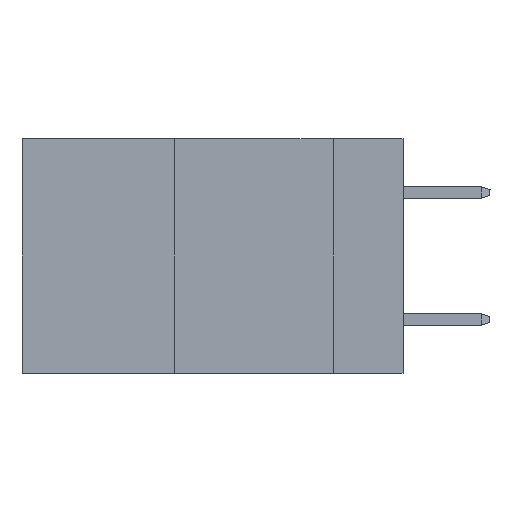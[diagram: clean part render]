
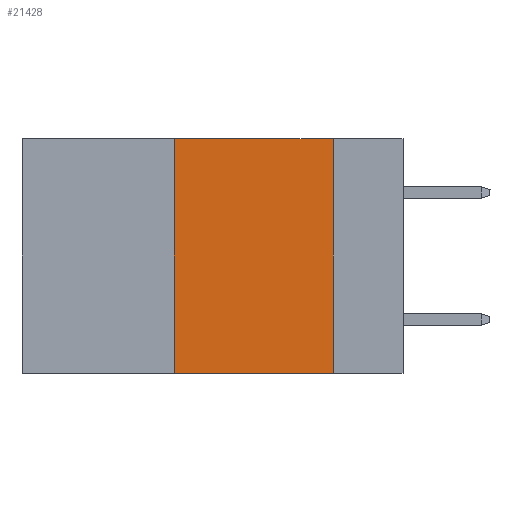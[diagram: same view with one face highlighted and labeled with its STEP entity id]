
A CAD part, left-side view. The second image highlights one B-rep face of the part: STEP entity #21428.
In plain terms, the highlighted planar face has unit normal (-1, 0, 0).
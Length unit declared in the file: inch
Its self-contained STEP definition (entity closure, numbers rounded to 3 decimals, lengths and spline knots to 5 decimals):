
#2972 = VERTEX_POINT ( 'NONE', #30787 ) ;
#3745 = VERTEX_POINT ( 'NONE', #15633 ) ;
#4530 = CARTESIAN_POINT ( 'NONE',  ( 0., 0.6, -0.37 ) ) ;
#4859 = CARTESIAN_POINT ( 'NONE',  ( 0., 0.6, 0. ) ) ;
#5499 = CARTESIAN_POINT ( 'NONE',  ( 0., 0.36, -0.37 ) ) ;
#5770 = ORIENTED_EDGE ( 'NONE', *, *, #16082, .F. ) ;
#7075 = FACE_OUTER_BOUND ( 'NONE', #10022, .T. ) ;
#7246 = LINE ( 'NONE', #9994, #15210 ) ;
#7948 = EDGE_CURVE ( 'NONE', #3745, #10744, #26972, .T. ) ;
#9994 = CARTESIAN_POINT ( 'NONE',  ( 0., 0.36, 0. ) ) ;
#10022 = EDGE_LOOP ( 'NONE', ( #14668, #28168, #5770, #11586 ) ) ;
#10233 = CARTESIAN_POINT ( 'NONE',  ( 0., 0.11, 0. ) ) ;
#10744 = VERTEX_POINT ( 'NONE', #10233 ) ;
#11127 = EDGE_CURVE ( 'NONE', #10744, #2972, #30096, .T. ) ;
#11586 = ORIENTED_EDGE ( 'NONE', *, *, #12188, .T. ) ;
#11981 = VECTOR ( 'NONE', #29694, 39.37008 ) ;
#12032 = DIRECTION ( 'NONE',  ( 0., 0., -1. ) ) ;
#12188 = EDGE_CURVE ( 'NONE', #24611, #2972, #30290, .T. ) ;
#13368 = VECTOR ( 'NONE', #22627, 39.37008 ) ;
#14284 = AXIS2_PLACEMENT_3D ( 'NONE', #4859, #30965, #14943 ) ;
#14584 = CARTESIAN_POINT ( 'NONE',  ( 0., 0.11, 0. ) ) ;
#14668 = ORIENTED_EDGE ( 'NONE', *, *, #11127, .F. ) ;
#14943 = DIRECTION ( 'NONE',  ( 0., 0., -1. ) ) ;
#15210 = VECTOR ( 'NONE', #24836, 39.37008 ) ;
#15283 = PLANE ( 'NONE',  #14284 ) ;
#15633 = CARTESIAN_POINT ( 'NONE',  ( 0., 0.36, 0. ) ) ;
#16082 = EDGE_CURVE ( 'NONE', #24611, #3745, #7246, .T. ) ;
#21428 = ADVANCED_FACE ( 'NONE', ( #7075 ), #15283, .F. ) ;
#22627 = DIRECTION ( 'NONE',  ( 0., -1., 0. ) ) ;
#24221 = VECTOR ( 'NONE', #12032, 39.37008 ) ;
#24260 = CARTESIAN_POINT ( 'NONE',  ( 0., 0.6, 0. ) ) ;
#24611 = VERTEX_POINT ( 'NONE', #5499 ) ;
#24836 = DIRECTION ( 'NONE',  ( 0., 0., 1. ) ) ;
#26972 = LINE ( 'NONE', #24260, #11981 ) ;
#28168 = ORIENTED_EDGE ( 'NONE', *, *, #7948, .F. ) ;
#29694 = DIRECTION ( 'NONE',  ( 0., -1., 0. ) ) ;
#30096 = LINE ( 'NONE', #14584, #24221 ) ;
#30290 = LINE ( 'NONE', #4530, #13368 ) ;
#30787 = CARTESIAN_POINT ( 'NONE',  ( 0., 0.11, -0.37 ) ) ;
#30965 = DIRECTION ( 'NONE',  ( 1., 0., 0. ) ) ;
